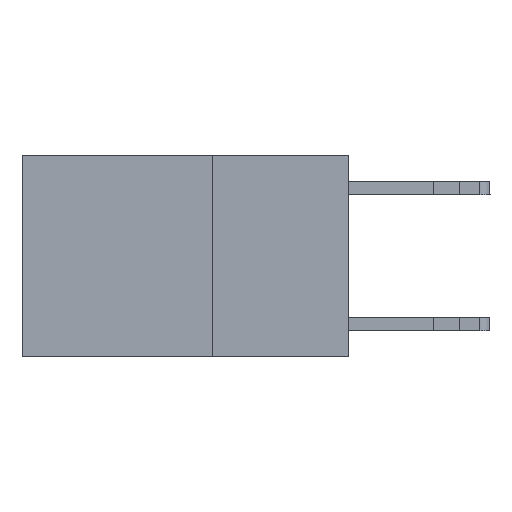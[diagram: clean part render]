
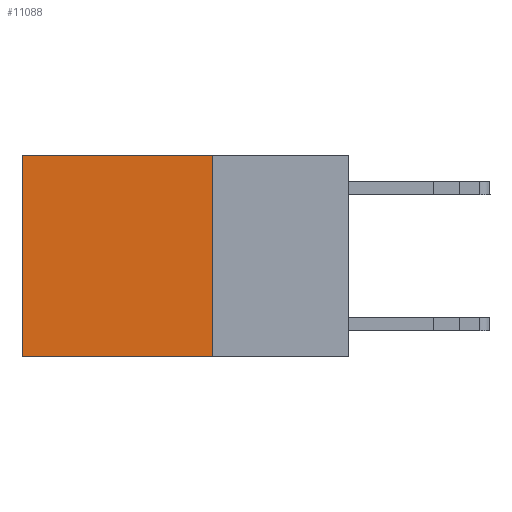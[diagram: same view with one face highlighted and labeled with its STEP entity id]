
A CAD part, left-side view. The second image highlights one B-rep face of the part: STEP entity #11088.
In plain terms, the highlighted planar face has unit normal (-1, 0, 0).
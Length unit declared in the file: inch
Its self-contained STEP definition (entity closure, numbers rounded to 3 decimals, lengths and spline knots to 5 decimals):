
#448 = CARTESIAN_POINT ( 'NONE',  ( 0.2625, 0.6, -0.37 ) ) ;
#593 = LINE ( 'NONE', #3646, #7738 ) ;
#1766 = VECTOR ( 'NONE', #4031, 39.37008 ) ;
#2989 = EDGE_LOOP ( 'NONE', ( #12245, #11983, #12344, #12262 ) ) ;
#3486 = DIRECTION ( 'NONE',  ( 0., 0., -1. ) ) ;
#3646 = CARTESIAN_POINT ( 'NONE',  ( 0.2625, 0.25, 0. ) ) ;
#4031 = DIRECTION ( 'NONE',  ( 0., 1., 0. ) ) ;
#5019 = FACE_OUTER_BOUND ( 'NONE', #2989, .T. ) ;
#6200 = DIRECTION ( 'NONE',  ( 0., 0., -1. ) ) ;
#6391 = DIRECTION ( 'NONE',  ( 0., 1., 0. ) ) ;
#6695 = CARTESIAN_POINT ( 'NONE',  ( 0.2625, 0.25, 0. ) ) ;
#6911 = LINE ( 'NONE', #11592, #16807 ) ;
#7738 = VECTOR ( 'NONE', #11609, 39.37008 ) ;
#7863 = CARTESIAN_POINT ( 'NONE',  ( 0.2625, 0.25, -0.37 ) ) ;
#8135 = VERTEX_POINT ( 'NONE', #448 ) ;
#8525 = EDGE_CURVE ( 'NONE', #9241, #12741, #14926, .T. ) ;
#8810 = CARTESIAN_POINT ( 'NONE',  ( 0.2625, 0.25, 0. ) ) ;
#9241 = VERTEX_POINT ( 'NONE', #6695 ) ;
#9459 = CARTESIAN_POINT ( 'NONE',  ( 0.2625, 0.6, 0. ) ) ;
#11088 = ADVANCED_FACE ( 'NONE', ( #5019 ), #16520, .F. ) ;
#11170 = EDGE_CURVE ( 'NONE', #9241, #11323, #593, .T. ) ;
#11323 = VERTEX_POINT ( 'NONE', #7863 ) ;
#11429 = VECTOR ( 'NONE', #6200, 39.37008 ) ;
#11460 = DIRECTION ( 'NONE',  ( 1., 0., 0. ) ) ;
#11471 = CARTESIAN_POINT ( 'NONE',  ( 0.2625, 0.6, 0. ) ) ;
#11592 = CARTESIAN_POINT ( 'NONE',  ( 0.2625, 0.25, -0.37 ) ) ;
#11609 = DIRECTION ( 'NONE',  ( 0., 0., -1. ) ) ;
#11951 = EDGE_CURVE ( 'NONE', #11323, #8135, #6911, .T. ) ;
#11961 = CARTESIAN_POINT ( 'NONE',  ( 0.2625, 0.25, 0. ) ) ;
#11983 = ORIENTED_EDGE ( 'NONE', *, *, #11951, .F. ) ;
#12245 = ORIENTED_EDGE ( 'NONE', *, *, #14614, .T. ) ;
#12262 = ORIENTED_EDGE ( 'NONE', *, *, #8525, .T. ) ;
#12344 = ORIENTED_EDGE ( 'NONE', *, *, #11170, .F. ) ;
#12494 = AXIS2_PLACEMENT_3D ( 'NONE', #8810, #11460, #3486 ) ;
#12741 = VERTEX_POINT ( 'NONE', #9459 ) ;
#14614 = EDGE_CURVE ( 'NONE', #12741, #8135, #14799, .T. ) ;
#14799 = LINE ( 'NONE', #11471, #11429 ) ;
#14926 = LINE ( 'NONE', #11961, #1766 ) ;
#16520 = PLANE ( 'NONE',  #12494 ) ;
#16807 = VECTOR ( 'NONE', #6391, 39.37008 ) ;
